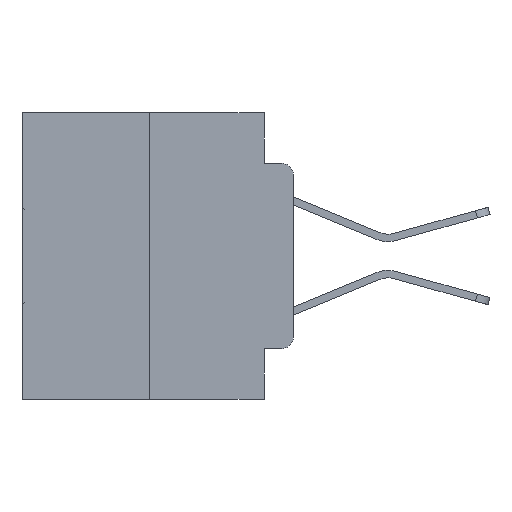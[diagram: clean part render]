
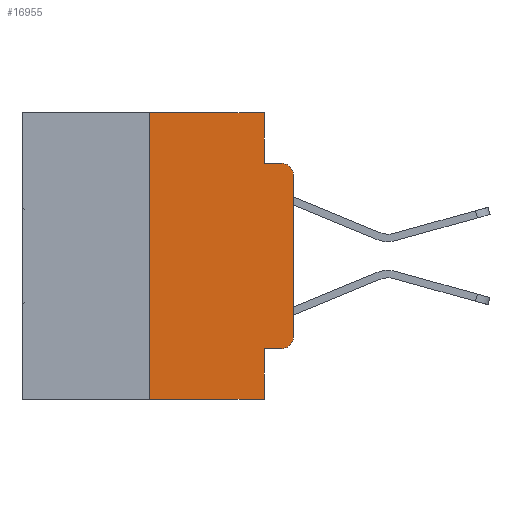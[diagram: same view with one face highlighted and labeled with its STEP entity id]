
A CAD part, left-side view. The second image highlights one B-rep face of the part: STEP entity #16955.
In plain terms, the highlighted planar face has unit normal (-1, 0, 0).
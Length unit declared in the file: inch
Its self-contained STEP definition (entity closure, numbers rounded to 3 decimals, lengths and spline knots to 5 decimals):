
#527 = LINE ( 'NONE', #997, #24622 ) ;
#674 = DIRECTION ( 'NONE',  ( 0., -1., 0. ) ) ;
#793 = EDGE_CURVE ( 'NONE', #19787, #10875, #5489, .T. ) ;
#997 = CARTESIAN_POINT ( 'NONE',  ( 0., 0., 0. ) ) ;
#1346 = LINE ( 'NONE', #7197, #2425 ) ;
#1543 = CARTESIAN_POINT ( 'NONE',  ( 0., 0., -0.3915 ) ) ;
#1671 = LINE ( 'NONE', #21186, #26465 ) ;
#1853 = DIRECTION ( 'NONE',  ( 0., 0., -1. ) ) ;
#2081 = ORIENTED_EDGE ( 'NONE', *, *, #24653, .F. ) ;
#2418 = EDGE_CURVE ( 'NONE', #19708, #7219, #1346, .T. ) ;
#2425 = VECTOR ( 'NONE', #26143, 39.37008 ) ;
#2973 = EDGE_CURVE ( 'NONE', #19308, #19787, #1671, .T. ) ;
#3686 = EDGE_CURVE ( 'NONE', #19308, #7219, #26059, .T. ) ;
#4099 = LINE ( 'NONE', #17325, #23443 ) ;
#4209 = CARTESIAN_POINT ( 'NONE',  ( 0., 0.051, -0.5 ) ) ;
#4215 = FACE_OUTER_BOUND ( 'NONE', #17784, .T. ) ;
#4765 = CARTESIAN_POINT ( 'NONE',  ( 0., 0.25, -0.5 ) ) ;
#5002 = CARTESIAN_POINT ( 'NONE',  ( 0., 0.051, -0.4115 ) ) ;
#5147 = VERTEX_POINT ( 'NONE', #5461 ) ;
#5277 = ORIENTED_EDGE ( 'NONE', *, *, #3686, .F. ) ;
#5461 = CARTESIAN_POINT ( 'NONE',  ( 0., 0.02, -0.0885 ) ) ;
#5489 = CIRCLE ( 'NONE', #15435, 0.02 ) ;
#5983 = ORIENTED_EDGE ( 'NONE', *, *, #13483, .F. ) ;
#6257 = DIRECTION ( 'NONE',  ( -1., 0., 0. ) ) ;
#6378 = DIRECTION ( 'NONE',  ( 0., 0., -1. ) ) ;
#6549 = DIRECTION ( 'NONE',  ( 0., 0., -1. ) ) ;
#6666 = ORIENTED_EDGE ( 'NONE', *, *, #21780, .T. ) ;
#6671 = PLANE ( 'NONE',  #8814 ) ;
#7197 = CARTESIAN_POINT ( 'NONE',  ( 0., 0.473, -0.5 ) ) ;
#7219 = VERTEX_POINT ( 'NONE', #4209 ) ;
#8532 = VERTEX_POINT ( 'NONE', #9675 ) ;
#8814 = AXIS2_PLACEMENT_3D ( 'NONE', #25421, #25222, #18383 ) ;
#9675 = CARTESIAN_POINT ( 'NONE',  ( 0., 0.051, 0. ) ) ;
#10263 = DIRECTION ( 'NONE',  ( 0., 0., 1. ) ) ;
#10429 = DIRECTION ( 'NONE',  ( 0., 0., -1. ) ) ;
#10644 = DIRECTION ( 'NONE',  ( -1., 0., 0. ) ) ;
#10875 = VERTEX_POINT ( 'NONE', #1543 ) ;
#10953 = CARTESIAN_POINT ( 'NONE',  ( 0., 0.02, -0.3915 ) ) ;
#11042 = ORIENTED_EDGE ( 'NONE', *, *, #25685, .F. ) ;
#11291 = CARTESIAN_POINT ( 'NONE',  ( 0., 0.051, -0.0885 ) ) ;
#11853 = CARTESIAN_POINT ( 'NONE',  ( 0., 0.051, -0.0885 ) ) ;
#12272 = ORIENTED_EDGE ( 'NONE', *, *, #793, .T. ) ;
#13248 = CIRCLE ( 'NONE', #23105, 0.02 ) ;
#13483 = EDGE_CURVE ( 'NONE', #8532, #22743, #27739, .T. ) ;
#13590 = CARTESIAN_POINT ( 'NONE',  ( 0., 0.02, -0.1085 ) ) ;
#15416 = VERTEX_POINT ( 'NONE', #21911 ) ;
#15435 = AXIS2_PLACEMENT_3D ( 'NONE', #10953, #10644, #6378 ) ;
#16299 = ORIENTED_EDGE ( 'NONE', *, *, #23651, .F. ) ;
#16594 = CARTESIAN_POINT ( 'NONE',  ( 0., 0., -0.1085 ) ) ;
#16955 = ADVANCED_FACE ( 'NONE', ( #4215 ), #6671, .F. ) ;
#17093 = CARTESIAN_POINT ( 'NONE',  ( 0., 0.25, 0. ) ) ;
#17325 = CARTESIAN_POINT ( 'NONE',  ( 0., 0.473, 0. ) ) ;
#17784 = EDGE_LOOP ( 'NONE', ( #6666, #20292, #11042, #5983, #16299, #2081, #27840, #5277, #25582, #12272 ) ) ;
#18058 = VECTOR ( 'NONE', #28117, 39.37008 ) ;
#18383 = DIRECTION ( 'NONE',  ( 0., 0., -1. ) ) ;
#18412 = VECTOR ( 'NONE', #6549, 39.37008 ) ;
#19308 = VERTEX_POINT ( 'NONE', #5002 ) ;
#19708 = VERTEX_POINT ( 'NONE', #4765 ) ;
#19717 = VECTOR ( 'NONE', #10429, 39.37008 ) ;
#19787 = VERTEX_POINT ( 'NONE', #23912 ) ;
#20292 = ORIENTED_EDGE ( 'NONE', *, *, #23309, .T. ) ;
#21186 = CARTESIAN_POINT ( 'NONE',  ( 0., 0.051, -0.4115 ) ) ;
#21780 = EDGE_CURVE ( 'NONE', #10875, #22280, #527, .T. ) ;
#21911 = CARTESIAN_POINT ( 'NONE',  ( 0., 0.25, 0. ) ) ;
#21992 = DIRECTION ( 'NONE',  ( 0., 0., 1. ) ) ;
#22280 = VERTEX_POINT ( 'NONE', #16594 ) ;
#22743 = VERTEX_POINT ( 'NONE', #11291 ) ;
#23105 = AXIS2_PLACEMENT_3D ( 'NONE', #13590, #6257, #1853 ) ;
#23309 = EDGE_CURVE ( 'NONE', #22280, #5147, #13248, .T. ) ;
#23443 = VECTOR ( 'NONE', #24154, 39.37008 ) ;
#23651 = EDGE_CURVE ( 'NONE', #15416, #8532, #4099, .T. ) ;
#23912 = CARTESIAN_POINT ( 'NONE',  ( 0., 0.02, -0.4115 ) ) ;
#24154 = DIRECTION ( 'NONE',  ( 0., -1., 0. ) ) ;
#24622 = VECTOR ( 'NONE', #21992, 39.37008 ) ;
#24653 = EDGE_CURVE ( 'NONE', #19708, #15416, #29785, .T. ) ;
#25222 = DIRECTION ( 'NONE',  ( 1., 0., 0. ) ) ;
#25421 = CARTESIAN_POINT ( 'NONE',  ( 0., 0.473, 0. ) ) ;
#25582 = ORIENTED_EDGE ( 'NONE', *, *, #2973, .T. ) ;
#25685 = EDGE_CURVE ( 'NONE', #22743, #5147, #26437, .T. ) ;
#26059 = LINE ( 'NONE', #29875, #18412 ) ;
#26143 = DIRECTION ( 'NONE',  ( 0., -1., 0. ) ) ;
#26437 = LINE ( 'NONE', #11853, #18058 ) ;
#26465 = VECTOR ( 'NONE', #674, 39.37008 ) ;
#27026 = CARTESIAN_POINT ( 'NONE',  ( 0., 0.051, 0. ) ) ;
#27739 = LINE ( 'NONE', #27026, #19717 ) ;
#27840 = ORIENTED_EDGE ( 'NONE', *, *, #2418, .T. ) ;
#28117 = DIRECTION ( 'NONE',  ( 0., -1., 0. ) ) ;
#29785 = LINE ( 'NONE', #17093, #30167 ) ;
#29875 = CARTESIAN_POINT ( 'NONE',  ( 0., 0.051, 0. ) ) ;
#30167 = VECTOR ( 'NONE', #10263, 39.37008 ) ;
